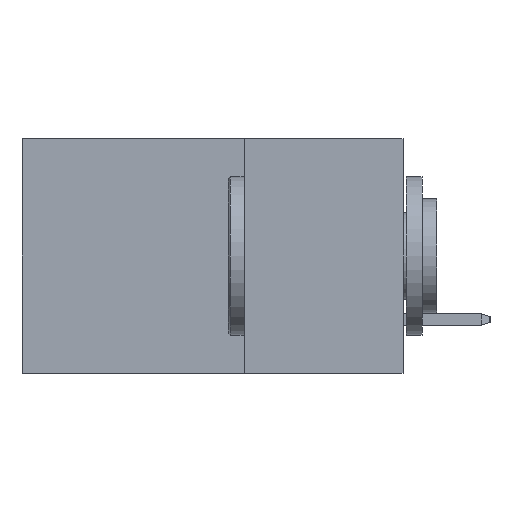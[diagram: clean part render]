
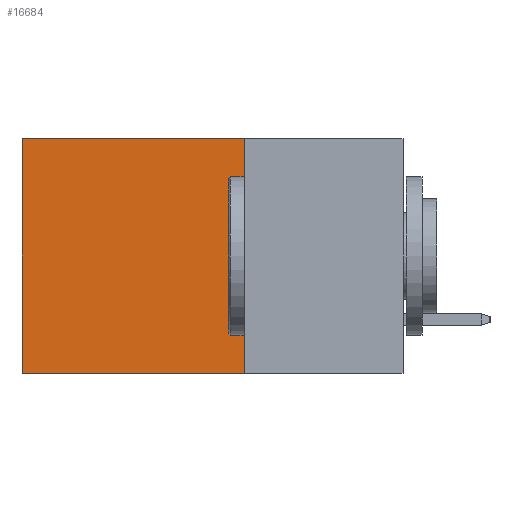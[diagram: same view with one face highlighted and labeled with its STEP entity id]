
A CAD part, left-side view. The second image highlights one B-rep face of the part: STEP entity #16684.
In plain terms, the highlighted planar face has unit normal (-1, 0, 0).
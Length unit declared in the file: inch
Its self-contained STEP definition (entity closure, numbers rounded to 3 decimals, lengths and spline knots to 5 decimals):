
#719 = DIRECTION ( 'NONE',  ( 1., 0., 0. ) ) ;
#1435 = CARTESIAN_POINT ( 'NONE',  ( 0.2875, 0.25, -0.37 ) ) ;
#1803 = LINE ( 'NONE', #10308, #18320 ) ;
#1855 = CARTESIAN_POINT ( 'NONE',  ( 0.2875, 0.25, -0.37 ) ) ;
#2342 = VERTEX_POINT ( 'NONE', #6913 ) ;
#2759 = CARTESIAN_POINT ( 'NONE',  ( 0.2875, 0.25, 0. ) ) ;
#3110 = CARTESIAN_POINT ( 'NONE',  ( 0.2875, 0.6, 0. ) ) ;
#3969 = CARTESIAN_POINT ( 'NONE',  ( 0.2875, 0.25, 0. ) ) ;
#5583 = VECTOR ( 'NONE', #9657, 39.37008 ) ;
#5977 = DIRECTION ( 'NONE',  ( 0., 1., 0. ) ) ;
#6079 = VERTEX_POINT ( 'NONE', #3110 ) ;
#6476 = DIRECTION ( 'NONE',  ( 0., 0., -1. ) ) ;
#6818 = DIRECTION ( 'NONE',  ( 0., 0., -1. ) ) ;
#6913 = CARTESIAN_POINT ( 'NONE',  ( 0.2875, 0.6, -0.37 ) ) ;
#7083 = EDGE_CURVE ( 'NONE', #10563, #6079, #14912, .T. ) ;
#7173 = LINE ( 'NONE', #1435, #5583 ) ;
#7430 = EDGE_CURVE ( 'NONE', #8340, #2342, #7173, .T. ) ;
#7792 = CARTESIAN_POINT ( 'NONE',  ( 0.2875, 0.25, 0. ) ) ;
#8340 = VERTEX_POINT ( 'NONE', #1855 ) ;
#8944 = EDGE_CURVE ( 'NONE', #10563, #8340, #10030, .T. ) ;
#9408 = FACE_OUTER_BOUND ( 'NONE', #17495, .T. ) ;
#9596 = PLANE ( 'NONE',  #13459 ) ;
#9657 = DIRECTION ( 'NONE',  ( 0., 1., 0. ) ) ;
#10030 = LINE ( 'NONE', #2759, #14128 ) ;
#10308 = CARTESIAN_POINT ( 'NONE',  ( 0.2875, 0.6, 0. ) ) ;
#10445 = ORIENTED_EDGE ( 'NONE', *, *, #7430, .F. ) ;
#10563 = VERTEX_POINT ( 'NONE', #3969 ) ;
#11585 = ORIENTED_EDGE ( 'NONE', *, *, #8944, .F. ) ;
#11934 = DIRECTION ( 'NONE',  ( 0., 0., -1. ) ) ;
#13459 = AXIS2_PLACEMENT_3D ( 'NONE', #7792, #719, #6476 ) ;
#14128 = VECTOR ( 'NONE', #6818, 39.37008 ) ;
#14340 = ORIENTED_EDGE ( 'NONE', *, *, #7083, .T. ) ;
#14726 = CARTESIAN_POINT ( 'NONE',  ( 0.2875, 0.25, 0. ) ) ;
#14912 = LINE ( 'NONE', #14726, #15944 ) ;
#15550 = ORIENTED_EDGE ( 'NONE', *, *, #17283, .T. ) ;
#15944 = VECTOR ( 'NONE', #5977, 39.37008 ) ;
#16684 = ADVANCED_FACE ( 'NONE', ( #9408 ), #9596, .F. ) ;
#17283 = EDGE_CURVE ( 'NONE', #6079, #2342, #1803, .T. ) ;
#17495 = EDGE_LOOP ( 'NONE', ( #15550, #10445, #11585, #14340 ) ) ;
#18320 = VECTOR ( 'NONE', #11934, 39.37008 ) ;
